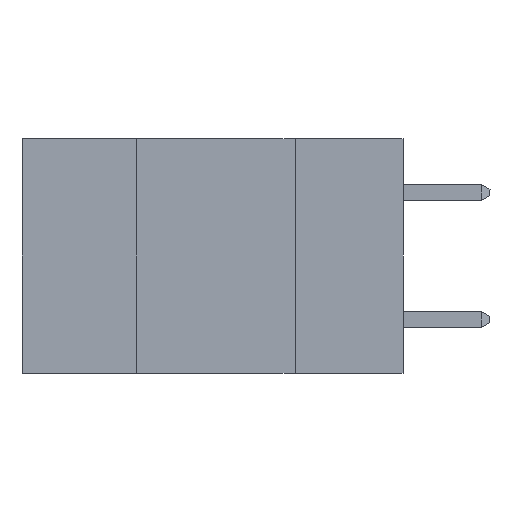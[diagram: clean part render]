
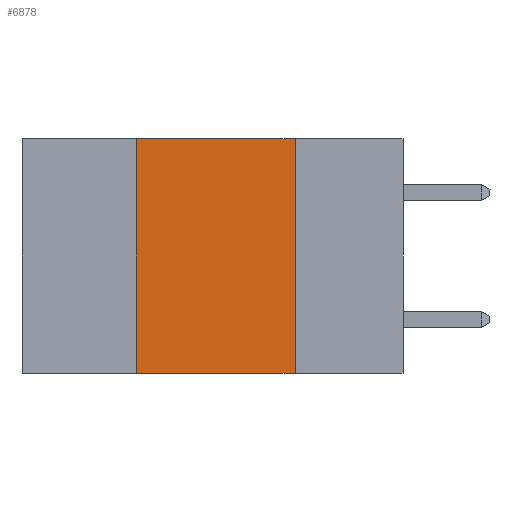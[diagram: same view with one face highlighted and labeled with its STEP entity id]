
A CAD part, left-side view. The second image highlights one B-rep face of the part: STEP entity #6878.
In plain terms, the highlighted planar face has unit normal (-1, 0, 0).
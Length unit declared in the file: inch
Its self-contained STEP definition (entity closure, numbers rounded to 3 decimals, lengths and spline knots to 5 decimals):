
#17 = VERTEX_POINT ( 'NONE', #10678 ) ;
#161 = ORIENTED_EDGE ( 'NONE', *, *, #10433, .F. ) ;
#286 = CARTESIAN_POINT ( 'NONE',  ( 0., 0.17, -0.37 ) ) ;
#486 = DIRECTION ( 'NONE',  ( 1., 0., 0. ) ) ;
#504 = VECTOR ( 'NONE', #10878, 39.37008 ) ;
#1217 = VERTEX_POINT ( 'NONE', #286 ) ;
#1391 = DIRECTION ( 'NONE',  ( 0., 0., 1. ) ) ;
#1836 = DIRECTION ( 'NONE',  ( 0., -1., 0. ) ) ;
#2006 = CARTESIAN_POINT ( 'NONE',  ( 0., 0.6, -0.37 ) ) ;
#2325 = DIRECTION ( 'NONE',  ( 0., 0., -1. ) ) ;
#2549 = CARTESIAN_POINT ( 'NONE',  ( 0., 0.42, 0. ) ) ;
#2874 = VECTOR ( 'NONE', #2325, 39.37008 ) ;
#2879 = VECTOR ( 'NONE', #1836, 39.37008 ) ;
#4110 = CARTESIAN_POINT ( 'NONE',  ( 0., 0.42, 0. ) ) ;
#4431 = DIRECTION ( 'NONE',  ( 0., 0., -1. ) ) ;
#4705 = EDGE_LOOP ( 'NONE', ( #161, #9297, #5112, #10260 ) ) ;
#4741 = VERTEX_POINT ( 'NONE', #12642 ) ;
#5112 = ORIENTED_EDGE ( 'NONE', *, *, #7745, .F. ) ;
#5386 = CARTESIAN_POINT ( 'NONE',  ( 0., 0.17, 0. ) ) ;
#6062 = VERTEX_POINT ( 'NONE', #4110 ) ;
#6558 = CARTESIAN_POINT ( 'NONE',  ( 0., 0.6, 0. ) ) ;
#6750 = AXIS2_PLACEMENT_3D ( 'NONE', #6558, #486, #4431 ) ;
#6878 = ADVANCED_FACE ( 'NONE', ( #12503 ), #9488, .F. ) ;
#6896 = LINE ( 'NONE', #11758, #504 ) ;
#7247 = LINE ( 'NONE', #2006, #2879 ) ;
#7745 = EDGE_CURVE ( 'NONE', #17, #6062, #11249, .T. ) ;
#7868 = LINE ( 'NONE', #5386, #2874 ) ;
#9297 = ORIENTED_EDGE ( 'NONE', *, *, #11241, .F. ) ;
#9488 = PLANE ( 'NONE',  #6750 ) ;
#10260 = ORIENTED_EDGE ( 'NONE', *, *, #12896, .T. ) ;
#10433 = EDGE_CURVE ( 'NONE', #4741, #1217, #7868, .T. ) ;
#10678 = CARTESIAN_POINT ( 'NONE',  ( 0., 0.42, -0.37 ) ) ;
#10878 = DIRECTION ( 'NONE',  ( 0., -1., 0. ) ) ;
#11241 = EDGE_CURVE ( 'NONE', #6062, #4741, #6896, .T. ) ;
#11249 = LINE ( 'NONE', #2549, #11880 ) ;
#11758 = CARTESIAN_POINT ( 'NONE',  ( 0., 0.6, 0. ) ) ;
#11880 = VECTOR ( 'NONE', #1391, 39.37008 ) ;
#12503 = FACE_OUTER_BOUND ( 'NONE', #4705, .T. ) ;
#12642 = CARTESIAN_POINT ( 'NONE',  ( 0., 0.17, 0. ) ) ;
#12896 = EDGE_CURVE ( 'NONE', #17, #1217, #7247, .T. ) ;
